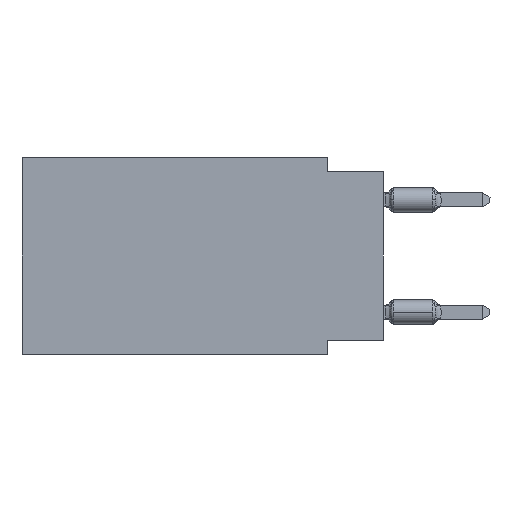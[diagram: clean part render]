
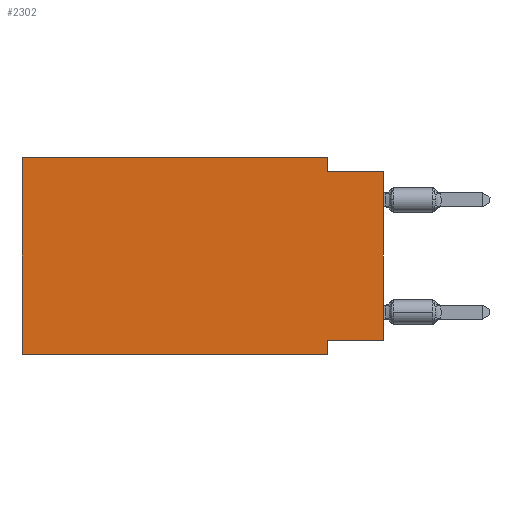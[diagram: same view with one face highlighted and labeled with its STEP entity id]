
A CAD part, left-side view. The second image highlights one B-rep face of the part: STEP entity #2302.
In plain terms, the highlighted planar face has unit normal (-1, 0, 0).
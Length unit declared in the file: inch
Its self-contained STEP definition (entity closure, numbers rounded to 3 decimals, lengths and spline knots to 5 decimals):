
#517 = LINE ( 'NONE', #7759, #1859 ) ;
#657 = VECTOR ( 'NONE', #21950, 39.37008 ) ;
#698 = VERTEX_POINT ( 'NONE', #10593 ) ;
#1184 = LINE ( 'NONE', #22382, #6230 ) ;
#1628 = CARTESIAN_POINT ( 'NONE',  ( 0., 0.645, 0. ) ) ;
#1670 = LINE ( 'NONE', #11266, #8589 ) ;
#1859 = VECTOR ( 'NONE', #6254, 39.37008 ) ;
#2302 = ADVANCED_FACE ( 'NONE', ( #18114 ), #7120, .F. ) ;
#3358 = ORIENTED_EDGE ( 'NONE', *, *, #12560, .F. ) ;
#3781 = DIRECTION ( 'NONE',  ( 0., -1., 0. ) ) ;
#3984 = EDGE_CURVE ( 'NONE', #9360, #23597, #15833, .T. ) ;
#4303 = CARTESIAN_POINT ( 'NONE',  ( 0., 0.1, -0.35 ) ) ;
#4834 = CARTESIAN_POINT ( 'NONE',  ( 0., 0., -0.325 ) ) ;
#5022 = LINE ( 'NONE', #24358, #12727 ) ;
#6230 = VECTOR ( 'NONE', #16147, 39.37008 ) ;
#6254 = DIRECTION ( 'NONE',  ( 0., 0., 1. ) ) ;
#7120 = PLANE ( 'NONE',  #17008 ) ;
#7256 = CARTESIAN_POINT ( 'NONE',  ( 0., 0.1, 0. ) ) ;
#7357 = VERTEX_POINT ( 'NONE', #4834 ) ;
#7759 = CARTESIAN_POINT ( 'NONE',  ( 0., 0.645, 0. ) ) ;
#8581 = VECTOR ( 'NONE', #21821, 39.37008 ) ;
#8589 = VECTOR ( 'NONE', #3781, 39.37008 ) ;
#9166 = VERTEX_POINT ( 'NONE', #4303 ) ;
#9360 = VERTEX_POINT ( 'NONE', #9527 ) ;
#9527 = CARTESIAN_POINT ( 'NONE',  ( 0., 0.645, 0. ) ) ;
#9872 = EDGE_CURVE ( 'NONE', #23597, #23501, #18854, .T. ) ;
#9979 = CARTESIAN_POINT ( 'NONE',  ( 0., 0.645, 0. ) ) ;
#10473 = ORIENTED_EDGE ( 'NONE', *, *, #20780, .T. ) ;
#10589 = CARTESIAN_POINT ( 'NONE',  ( 0., 0.1, -0.35 ) ) ;
#10593 = CARTESIAN_POINT ( 'NONE',  ( 0., 0.645, -0.35 ) ) ;
#11095 = CARTESIAN_POINT ( 'NONE',  ( 0., 0., -0.025 ) ) ;
#11228 = EDGE_CURVE ( 'NONE', #698, #9166, #1670, .T. ) ;
#11266 = CARTESIAN_POINT ( 'NONE',  ( 0., 0.645, -0.35 ) ) ;
#11818 = EDGE_CURVE ( 'NONE', #15684, #9166, #14458, .T. ) ;
#12108 = VERTEX_POINT ( 'NONE', #18166 ) ;
#12560 = EDGE_CURVE ( 'NONE', #23501, #12108, #13102, .T. ) ;
#12727 = VECTOR ( 'NONE', #22003, 39.37008 ) ;
#12855 = DIRECTION ( 'NONE',  ( 1., 0., 0. ) ) ;
#13102 = LINE ( 'NONE', #11095, #16205 ) ;
#14458 = LINE ( 'NONE', #10589, #657 ) ;
#15684 = VERTEX_POINT ( 'NONE', #17429 ) ;
#15833 = LINE ( 'NONE', #9979, #8581 ) ;
#16147 = DIRECTION ( 'NONE',  ( 0., 0., 1. ) ) ;
#16205 = VECTOR ( 'NONE', #22336, 39.37008 ) ;
#17008 = AXIS2_PLACEMENT_3D ( 'NONE', #1628, #12855, #21977 ) ;
#17429 = CARTESIAN_POINT ( 'NONE',  ( 0., 0.1, -0.325 ) ) ;
#17474 = EDGE_CURVE ( 'NONE', #7357, #15684, #5022, .T. ) ;
#17482 = ORIENTED_EDGE ( 'NONE', *, *, #9872, .F. ) ;
#18038 = ORIENTED_EDGE ( 'NONE', *, *, #11228, .T. ) ;
#18114 = FACE_OUTER_BOUND ( 'NONE', #22970, .T. ) ;
#18166 = CARTESIAN_POINT ( 'NONE',  ( 0., 0., -0.025 ) ) ;
#18406 = ORIENTED_EDGE ( 'NONE', *, *, #21419, .F. ) ;
#18854 = LINE ( 'NONE', #7256, #19979 ) ;
#19979 = VECTOR ( 'NONE', #20730, 39.37008 ) ;
#20730 = DIRECTION ( 'NONE',  ( 0., 0., -1. ) ) ;
#20780 = EDGE_CURVE ( 'NONE', #7357, #12108, #1184, .T. ) ;
#21162 = CARTESIAN_POINT ( 'NONE',  ( 0., 0.1, -0.025 ) ) ;
#21419 = EDGE_CURVE ( 'NONE', #698, #9360, #517, .T. ) ;
#21821 = DIRECTION ( 'NONE',  ( 0., -1., 0. ) ) ;
#21950 = DIRECTION ( 'NONE',  ( 0., 0., -1. ) ) ;
#21977 = DIRECTION ( 'NONE',  ( 0., 0., -1. ) ) ;
#22003 = DIRECTION ( 'NONE',  ( 0., 1., 0. ) ) ;
#22336 = DIRECTION ( 'NONE',  ( 0., -1., 0. ) ) ;
#22382 = CARTESIAN_POINT ( 'NONE',  ( 0., 0., 0. ) ) ;
#22445 = ORIENTED_EDGE ( 'NONE', *, *, #11818, .F. ) ;
#22496 = CARTESIAN_POINT ( 'NONE',  ( 0., 0.1, 0. ) ) ;
#22970 = EDGE_LOOP ( 'NONE', ( #10473, #3358, #17482, #23292, #18406, #18038, #22445, #23185 ) ) ;
#23185 = ORIENTED_EDGE ( 'NONE', *, *, #17474, .F. ) ;
#23292 = ORIENTED_EDGE ( 'NONE', *, *, #3984, .F. ) ;
#23501 = VERTEX_POINT ( 'NONE', #21162 ) ;
#23597 = VERTEX_POINT ( 'NONE', #22496 ) ;
#24358 = CARTESIAN_POINT ( 'NONE',  ( 0., 0., -0.325 ) ) ;
